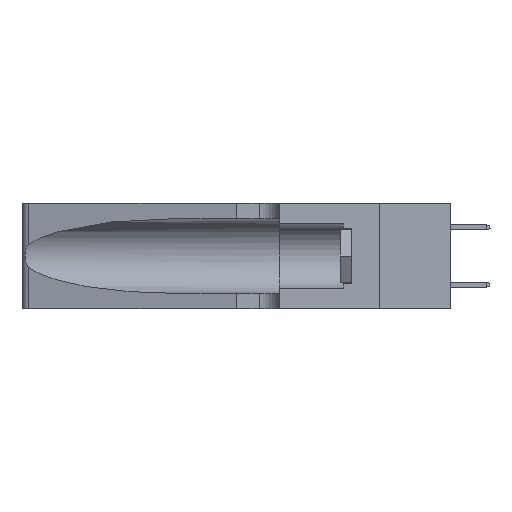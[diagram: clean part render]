
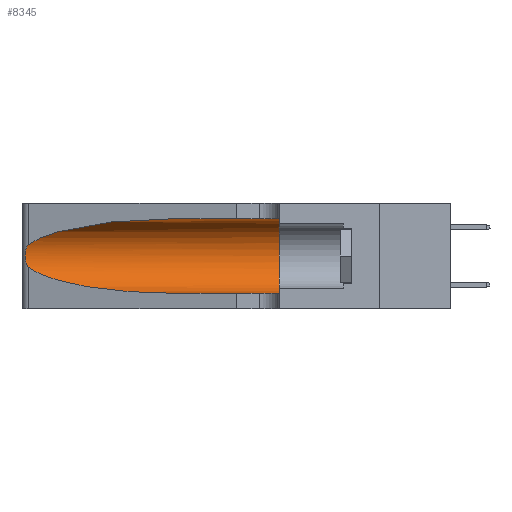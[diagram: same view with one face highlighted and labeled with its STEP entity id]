
A CAD part, left-side view. The second image highlights one B-rep face of the part: STEP entity #8345.
In plain terms, the highlighted cylindrical face has radius 3.308 mm (diameter 6.617 mm), a partial arc.
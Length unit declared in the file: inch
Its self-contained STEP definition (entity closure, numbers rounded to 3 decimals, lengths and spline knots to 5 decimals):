
#123 = B_SPLINE_CURVE_WITH_KNOTS ( 'NONE', 3,
 ( #5022, #30260, #2015, #24964, #33271, #30995, #33653, #4451, #7482, #16310, #13479, #36440, #22130, #7872 ),
 .UNSPECIFIED., .F., .F.,
 ( 4, 2, 2, 2, 2, 2, 4 ),
 ( 0., 0.00027, 0.00053, 0.00107, 0.0016, 0.00187, 0.00214 ),
 .UNSPECIFIED. ) ;
#511 = CIRCLE ( 'NONE', #22738, 0.13025 ) ;
#512 = CARTESIAN_POINT ( 'NONE',  ( 0.1305, 0.72297, 0.05475 ) ) ;
#1158 = VECTOR ( 'NONE', #32996, 39.37008 ) ;
#1999 = EDGE_CURVE ( 'NONE', #23964, #31400, #22168, .T. ) ;
#2015 = CARTESIAN_POINT ( 'NONE',  ( 0.25639, 1.23184, 0.21858 ) ) ;
#2905 = VERTEX_POINT ( 'NONE', #512 ) ;
#3187 = VERTEX_POINT ( 'NONE', #28186 ) ;
#3447 = CARTESIAN_POINT ( 'NONE',  ( 0.1305, 1.61858, 0.05475 ) ) ;
#3882 = CARTESIAN_POINT ( 'NONE',  ( 0.25487, 1.22718, 0.22369 ) ) ;
#4451 = CARTESIAN_POINT ( 'NONE',  ( 0.26075, 1.23896, 0.178 ) ) ;
#5022 = CARTESIAN_POINT ( 'NONE',  ( 0.25487, 1.22718, 0.22369 ) ) ;
#7482 = CARTESIAN_POINT ( 'NONE',  ( 0.26017, 1.23833, 0.17102 ) ) ;
#7872 = CARTESIAN_POINT ( 'NONE',  ( 0.25487, 1.22718, 0.14631 ) ) ;
#8295 = ORIENTED_EDGE ( 'NONE', *, *, #20622, .F. ) ;
#8345 = ADVANCED_FACE ( 'NONE', ( #16399 ), #24308, .F. ) ;
#8605 = CARTESIAN_POINT ( 'NONE',  ( 0.1305, 0.72297, 0.31525 ) ) ;
#8920 = DIRECTION ( 'NONE',  ( 0., -1., 0. ) ) ;
#9197 = ORIENTED_EDGE ( 'NONE', *, *, #21809, .T. ) ;
#10098 = EDGE_CURVE ( 'NONE', #2905, #3187, #29261, .T. ) ;
#10232 = DIRECTION ( 'NONE',  ( 0., 0., 1. ) ) ;
#11420 = CARTESIAN_POINT ( 'NONE',  ( 0.2373, 1.15595, 0.28018 ) ) ;
#12651 = CARTESIAN_POINT ( 'NONE',  ( 0.1305, 0.72297, 0.05475 ) ) ;
#12829 = CARTESIAN_POINT ( 'NONE',  ( 0.1305, 1.61858, 0.31525 ) ) ;
#13479 = CARTESIAN_POINT ( 'NONE',  ( 0.25789, 1.23486, 0.15765 ) ) ;
#14057 = CARTESIAN_POINT ( 'NONE',  ( 0.18966, 0.96281, 0.31525 ) ) ;
#15691 =( BOUNDED_CURVE ( )  B_SPLINE_CURVE ( 3, ( #26794, #18282, #32073, #12651 ),
 .UNSPECIFIED., .F., .T. ) 
 B_SPLINE_CURVE_WITH_KNOTS ( ( 4, 4 ),
 ( 3.44316, 4.71239 ),
 .UNSPECIFIED. ) 
 CURVE ( )  GEOMETRIC_REPRESENTATION_ITEM ( )  RATIONAL_B_SPLINE_CURVE ( ( 1., 0.87, 0.87, 1. ) ) 
 REPRESENTATION_ITEM ( '' )  );
#15760 = ORIENTED_EDGE ( 'NONE', *, *, #1999, .T. ) ;
#16310 = CARTESIAN_POINT ( 'NONE',  ( 0.25856, 1.23593, 0.16098 ) ) ;
#16398 = LINE ( 'NONE', #12829, #1158 ) ;
#16399 = FACE_OUTER_BOUND ( 'NONE', #21440, .T. ) ;
#17650 = EDGE_CURVE ( 'NONE', #23257, #3187, #511, .T. ) ;
#18282 = CARTESIAN_POINT ( 'NONE',  ( 0.2373, 1.15595, 0.08982 ) ) ;
#18855 = DIRECTION ( 'NONE',  ( 0., 0., -1. ) ) ;
#19669 = EDGE_CURVE ( 'NONE', #31400, #37114, #123, .T. ) ;
#20161 = CARTESIAN_POINT ( 'NONE',  ( 0.1305, 0.72297, 0.31525 ) ) ;
#20622 = EDGE_CURVE ( 'NONE', #23964, #23257, #16398, .T. ) ;
#21440 = EDGE_LOOP ( 'NONE', ( #15760, #35798, #9197, #23061, #31928, #8295 ) ) ;
#21809 = EDGE_CURVE ( 'NONE', #37114, #2905, #15691, .T. ) ;
#22130 = CARTESIAN_POINT ( 'NONE',  ( 0.25555, 1.22993, 0.14849 ) ) ;
#22168 =( BOUNDED_CURVE ( )  B_SPLINE_CURVE ( 3, ( #8605, #14057, #11420, #36664 ),
 .UNSPECIFIED., .F., .T. ) 
 B_SPLINE_CURVE_WITH_KNOTS ( ( 4, 4 ),
 ( 1.5708, 2.84003 ),
 .UNSPECIFIED. ) 
 CURVE ( )  GEOMETRIC_REPRESENTATION_ITEM ( )  RATIONAL_B_SPLINE_CURVE ( ( 1., 0.87, 0.87, 1. ) ) 
 REPRESENTATION_ITEM ( '' )  );
#22738 = AXIS2_PLACEMENT_3D ( 'NONE', #35996, #24892, #10232 ) ;
#23061 = ORIENTED_EDGE ( 'NONE', *, *, #10098, .T. ) ;
#23257 = VERTEX_POINT ( 'NONE', #36418 ) ;
#23964 = VERTEX_POINT ( 'NONE', #20161 ) ;
#24308 = CYLINDRICAL_SURFACE ( 'NONE', #33150, 0.13025 ) ;
#24892 = DIRECTION ( 'NONE',  ( 0., 1., 0. ) ) ;
#24964 = CARTESIAN_POINT ( 'NONE',  ( 0.25787, 1.23484, 0.2124 ) ) ;
#26013 = CARTESIAN_POINT ( 'NONE',  ( 0.25487, 1.22718, 0.14631 ) ) ;
#26619 = VECTOR ( 'NONE', #8920, 39.37008 ) ;
#26794 = CARTESIAN_POINT ( 'NONE',  ( 0.25487, 1.22718, 0.14631 ) ) ;
#27356 = CARTESIAN_POINT ( 'NONE',  ( 0.1305, 1.61858, 0.185 ) ) ;
#28186 = CARTESIAN_POINT ( 'NONE',  ( 0.1305, 0.35, 0.05475 ) ) ;
#29261 = LINE ( 'NONE', #3447, #26619 ) ;
#30260 = CARTESIAN_POINT ( 'NONE',  ( 0.25555, 1.22994, 0.2215 ) ) ;
#30995 = CARTESIAN_POINT ( 'NONE',  ( 0.26018, 1.23835, 0.19895 ) ) ;
#31400 = VERTEX_POINT ( 'NONE', #3882 ) ;
#31928 = ORIENTED_EDGE ( 'NONE', *, *, #17650, .F. ) ;
#32073 = CARTESIAN_POINT ( 'NONE',  ( 0.18966, 0.96281, 0.05475 ) ) ;
#32996 = DIRECTION ( 'NONE',  ( 0., -1., 0. ) ) ;
#33150 = AXIS2_PLACEMENT_3D ( 'NONE', #27356, #35784, #18855 ) ;
#33271 = CARTESIAN_POINT ( 'NONE',  ( 0.25854, 1.2359, 0.20912 ) ) ;
#33653 = CARTESIAN_POINT ( 'NONE',  ( 0.26075, 1.23896, 0.19203 ) ) ;
#35784 = DIRECTION ( 'NONE',  ( 0., -1., 0. ) ) ;
#35798 = ORIENTED_EDGE ( 'NONE', *, *, #19669, .T. ) ;
#35996 = CARTESIAN_POINT ( 'NONE',  ( 0.1305, 0.35, 0.185 ) ) ;
#36418 = CARTESIAN_POINT ( 'NONE',  ( 0.1305, 0.35, 0.31525 ) ) ;
#36440 = CARTESIAN_POINT ( 'NONE',  ( 0.25639, 1.23186, 0.15144 ) ) ;
#36664 = CARTESIAN_POINT ( 'NONE',  ( 0.25487, 1.22718, 0.22369 ) ) ;
#37114 = VERTEX_POINT ( 'NONE', #26013 ) ;
